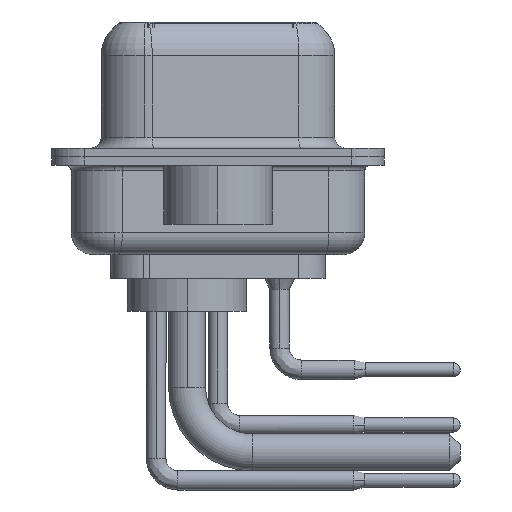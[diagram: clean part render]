
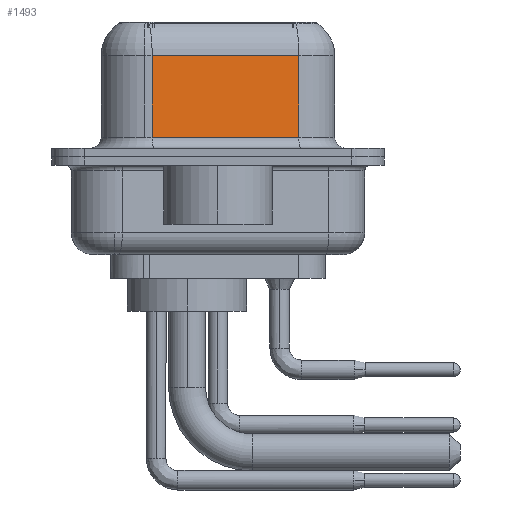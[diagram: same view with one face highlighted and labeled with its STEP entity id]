
A CAD part, left-side view. The second image highlights one B-rep face of the part: STEP entity #1493.
In plain terms, the highlighted planar face has unit normal (-0.985, -0.174, 0).
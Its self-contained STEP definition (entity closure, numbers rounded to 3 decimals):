
#874 = VERTEX_POINT ( 'NONE', #11380 ) ;
#1421 = EDGE_CURVE ( 'NONE', #12436, #874, #19576, .T. ) ;
#1493 = ADVANCED_FACE ( 'NONE', ( #7853 ), #28843, .F. ) ;
#1731 = CARTESIAN_POINT ( 'NONE',  ( 4.43, 3.028, 0.9 ) ) ;
#2804 = CARTESIAN_POINT ( 'NONE',  ( 5.621, -3.722, 0.9 ) ) ;
#5707 = CARTESIAN_POINT ( 'NONE',  ( 5.621, -3.722, 0.9 ) ) ;
#6053 = CARTESIAN_POINT ( 'NONE',  ( 5.621, -3.722, 6.4 ) ) ;
#7586 = LINE ( 'NONE', #10529, #33333 ) ;
#7853 = FACE_OUTER_BOUND ( 'NONE', #17703, .T. ) ;
#8458 = LINE ( 'NONE', #6053, #31343 ) ;
#9364 = ORIENTED_EDGE ( 'NONE', *, *, #22641, .T. ) ;
#10529 = CARTESIAN_POINT ( 'NONE',  ( 4.43, 3.028, 6.4 ) ) ;
#10586 = VERTEX_POINT ( 'NONE', #5707 ) ;
#11380 = CARTESIAN_POINT ( 'NONE',  ( 4.43, 3.028, 4.65 ) ) ;
#12436 = VERTEX_POINT ( 'NONE', #23108 ) ;
#12708 = VERTEX_POINT ( 'NONE', #1731 ) ;
#13934 = EDGE_CURVE ( 'NONE', #12436, #10586, #8458, .T. ) ;
#14091 = ORIENTED_EDGE ( 'NONE', *, *, #1421, .T. ) ;
#16018 = ORIENTED_EDGE ( 'NONE', *, *, #13934, .F. ) ;
#17703 = EDGE_LOOP ( 'NONE', ( #16018, #14091, #9364, #24369 ) ) ;
#18087 = VECTOR ( 'NONE', #31021, 1000. ) ;
#18633 = DIRECTION ( 'NONE',  ( 0., 0., -1. ) ) ;
#19576 = LINE ( 'NONE', #28003, #32605 ) ;
#20768 = CARTESIAN_POINT ( 'NONE',  ( 5.621, -3.722, 6.4 ) ) ;
#22170 = DIRECTION ( 'NONE',  ( -0.174, 0.985, 0. ) ) ;
#22641 = EDGE_CURVE ( 'NONE', #874, #12708, #7586, .T. ) ;
#23108 = CARTESIAN_POINT ( 'NONE',  ( 5.621, -3.722, 4.65 ) ) ;
#24369 = ORIENTED_EDGE ( 'NONE', *, *, #30975, .T. ) ;
#25696 = LINE ( 'NONE', #2804, #18087 ) ;
#26004 = AXIS2_PLACEMENT_3D ( 'NONE', #20768, #33505, #31424 ) ;
#28003 = CARTESIAN_POINT ( 'NONE',  ( 5.621, -3.722, 4.65 ) ) ;
#28759 = DIRECTION ( 'NONE',  ( 0., 0., -1. ) ) ;
#28843 = PLANE ( 'NONE',  #26004 ) ;
#30975 = EDGE_CURVE ( 'NONE', #12708, #10586, #25696, .T. ) ;
#31021 = DIRECTION ( 'NONE',  ( 0.174, -0.985, 0. ) ) ;
#31343 = VECTOR ( 'NONE', #18633, 1000. ) ;
#31424 = DIRECTION ( 'NONE',  ( -0.174, 0.985, 0. ) ) ;
#32605 = VECTOR ( 'NONE', #22170, 1000. ) ;
#33333 = VECTOR ( 'NONE', #28759, 1000. ) ;
#33505 = DIRECTION ( 'NONE',  ( 0.985, 0.174, 0. ) ) ;
